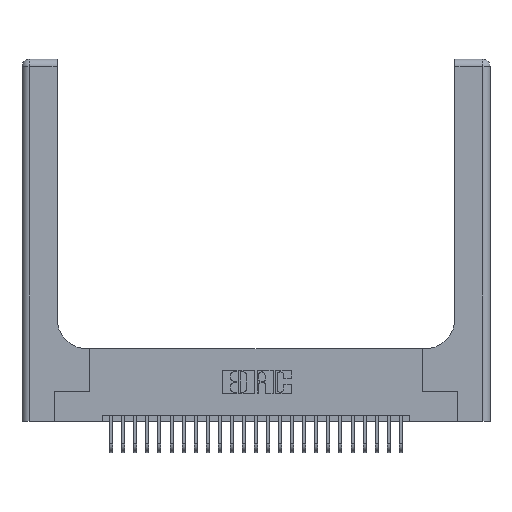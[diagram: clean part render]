
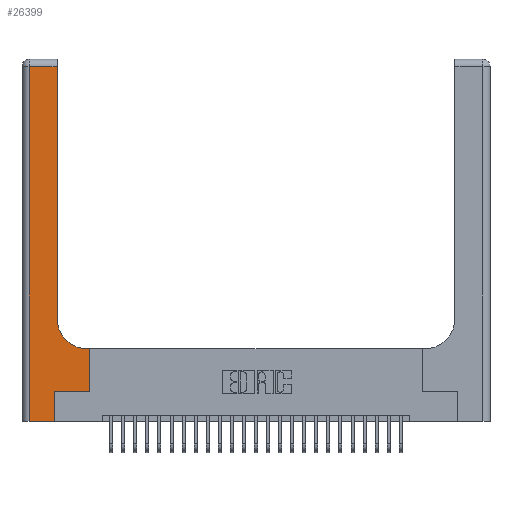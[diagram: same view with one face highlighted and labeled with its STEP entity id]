
A CAD part, top view. The second image highlights one B-rep face of the part: STEP entity #26399.
In plain terms, the highlighted planar face has unit normal (0, 0, 1).
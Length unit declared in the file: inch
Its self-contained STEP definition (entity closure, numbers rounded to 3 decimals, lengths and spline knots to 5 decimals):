
#130 = LINE ( 'NONE', #18337, #9779 ) ;
#624 = CARTESIAN_POINT ( 'NONE',  ( 0., 3., 0.37 ) ) ;
#1024 = DIRECTION ( 'NONE',  ( 1., 0., 0. ) ) ;
#1289 = CARTESIAN_POINT ( 'NONE',  ( 0.06, 3., 0.37 ) ) ;
#1351 = LINE ( 'NONE', #22300, #22436 ) ;
#1892 = AXIS2_PLACEMENT_3D ( 'NONE', #624, #14959, #2703 ) ;
#2339 = CARTESIAN_POINT ( 'NONE',  ( 0.269, 0.25, 0.37 ) ) ;
#2373 = LINE ( 'NONE', #24017, #7170 ) ;
#2567 = CARTESIAN_POINT ( 'NONE',  ( 0.2915, 0.6, 0.37 ) ) ;
#2703 = DIRECTION ( 'NONE',  ( -1., 0., 0. ) ) ;
#2859 = EDGE_CURVE ( 'NONE', #9038, #25445, #130, .T. ) ;
#2947 = ORIENTED_EDGE ( 'NONE', *, *, #8162, .T. ) ;
#5486 = DIRECTION ( 'NONE',  ( 0., 1., 0. ) ) ;
#5800 = CARTESIAN_POINT ( 'NONE',  ( 0.269, 0., 0.37 ) ) ;
#6219 = LINE ( 'NONE', #2567, #10977 ) ;
#6424 = EDGE_CURVE ( 'NONE', #18501, #6622, #8189, .T. ) ;
#6622 = VERTEX_POINT ( 'NONE', #5800 ) ;
#7157 = EDGE_CURVE ( 'NONE', #7432, #15122, #2373, .T. ) ;
#7170 = VECTOR ( 'NONE', #9840, 39.37008 ) ;
#7432 = VERTEX_POINT ( 'NONE', #14814 ) ;
#7445 = EDGE_CURVE ( 'NONE', #25445, #20118, #6219, .T. ) ;
#7953 = EDGE_CURVE ( 'NONE', #20118, #7432, #14473, .T. ) ;
#8162 = EDGE_CURVE ( 'NONE', #6622, #8502, #14780, .T. ) ;
#8189 = LINE ( 'NONE', #15272, #18387 ) ;
#8273 = DIRECTION ( 'NONE',  ( 0., 1., 0. ) ) ;
#8502 = VERTEX_POINT ( 'NONE', #2339 ) ;
#8821 = EDGE_CURVE ( 'NONE', #18992, #18501, #21074, .T. ) ;
#8905 = DIRECTION ( 'NONE',  ( 0., 0., -1. ) ) ;
#9038 = VERTEX_POINT ( 'NONE', #24461 ) ;
#9779 = VECTOR ( 'NONE', #8273, 39.37008 ) ;
#9840 = DIRECTION ( 'NONE',  ( 0., 1., 0. ) ) ;
#10318 = ORIENTED_EDGE ( 'NONE', *, *, #7953, .T. ) ;
#10433 = EDGE_LOOP ( 'NONE', ( #25190, #15740, #24280, #12554, #2947, #10959, #22416, #20212, #10318 ) ) ;
#10850 = PLANE ( 'NONE',  #1892 ) ;
#10959 = ORIENTED_EDGE ( 'NONE', *, *, #12442, .T. ) ;
#10977 = VECTOR ( 'NONE', #20926, 39.37008 ) ;
#11199 = CARTESIAN_POINT ( 'NONE',  ( 0.06, 2.94, 0.37 ) ) ;
#11290 = CARTESIAN_POINT ( 'NONE',  ( 0.5585, 0.6, 0.37 ) ) ;
#12442 = EDGE_CURVE ( 'NONE', #8502, #9038, #1351, .T. ) ;
#12554 = ORIENTED_EDGE ( 'NONE', *, *, #6424, .T. ) ;
#12890 = EDGE_CURVE ( 'NONE', #15122, #18992, #17657, .T. ) ;
#13016 = CARTESIAN_POINT ( 'NONE',  ( 0.5415, 0.6, 0.37 ) ) ;
#14473 = CIRCLE ( 'NONE', #25804, 0.25 ) ;
#14780 = LINE ( 'NONE', #17700, #25511 ) ;
#14814 = CARTESIAN_POINT ( 'NONE',  ( 0.2915, 0.85, 0.37 ) ) ;
#14959 = DIRECTION ( 'NONE',  ( 0., 0., -1. ) ) ;
#15122 = VERTEX_POINT ( 'NONE', #20248 ) ;
#15272 = CARTESIAN_POINT ( 'NONE',  ( 0., 0., 0.37 ) ) ;
#15641 = DIRECTION ( 'NONE',  ( 0., -1., 0. ) ) ;
#15740 = ORIENTED_EDGE ( 'NONE', *, *, #12890, .T. ) ;
#15792 = CARTESIAN_POINT ( 'NONE',  ( 0.06, 0., 0.37 ) ) ;
#15930 = FACE_OUTER_BOUND ( 'NONE', #10433, .T. ) ;
#16344 = VECTOR ( 'NONE', #15641, 39.37008 ) ;
#17657 = LINE ( 'NONE', #18673, #23670 ) ;
#17700 = CARTESIAN_POINT ( 'NONE',  ( 0.269, 0., 0.37 ) ) ;
#18337 = CARTESIAN_POINT ( 'NONE',  ( 0.5585, 0.25, 0.37 ) ) ;
#18387 = VECTOR ( 'NONE', #1024, 39.37008 ) ;
#18501 = VERTEX_POINT ( 'NONE', #15792 ) ;
#18673 = CARTESIAN_POINT ( 'NONE',  ( 0., 2.94, 0.37 ) ) ;
#18992 = VERTEX_POINT ( 'NONE', #11199 ) ;
#20118 = VERTEX_POINT ( 'NONE', #13016 ) ;
#20212 = ORIENTED_EDGE ( 'NONE', *, *, #7445, .T. ) ;
#20248 = CARTESIAN_POINT ( 'NONE',  ( 0.2915, 2.94, 0.37 ) ) ;
#20359 = DIRECTION ( 'NONE',  ( 1., 0., 0. ) ) ;
#20709 = DIRECTION ( 'NONE',  ( -1., 0., 0. ) ) ;
#20926 = DIRECTION ( 'NONE',  ( -1., 0., 0. ) ) ;
#21061 = CARTESIAN_POINT ( 'NONE',  ( 0.5415, 0.85, 0.37 ) ) ;
#21074 = LINE ( 'NONE', #1289, #16344 ) ;
#22300 = CARTESIAN_POINT ( 'NONE',  ( 0.269, 0.25, 0.37 ) ) ;
#22416 = ORIENTED_EDGE ( 'NONE', *, *, #2859, .T. ) ;
#22436 = VECTOR ( 'NONE', #20359, 39.37008 ) ;
#23105 = DIRECTION ( 'NONE',  ( 1., 0., 0. ) ) ;
#23670 = VECTOR ( 'NONE', #20709, 39.37008 ) ;
#24017 = CARTESIAN_POINT ( 'NONE',  ( 0.2915, 3., 0.37 ) ) ;
#24280 = ORIENTED_EDGE ( 'NONE', *, *, #8821, .T. ) ;
#24461 = CARTESIAN_POINT ( 'NONE',  ( 0.5585, 0.25, 0.37 ) ) ;
#25190 = ORIENTED_EDGE ( 'NONE', *, *, #7157, .T. ) ;
#25445 = VERTEX_POINT ( 'NONE', #11290 ) ;
#25511 = VECTOR ( 'NONE', #5486, 39.37008 ) ;
#25804 = AXIS2_PLACEMENT_3D ( 'NONE', #21061, #8905, #23105 ) ;
#26399 = ADVANCED_FACE ( 'NONE', ( #15930 ), #10850, .F. ) ;
